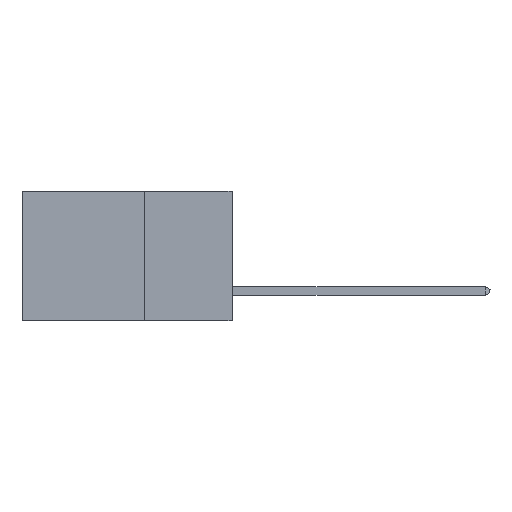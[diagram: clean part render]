
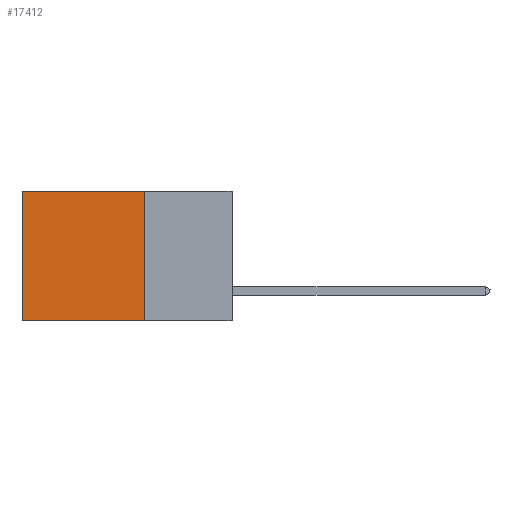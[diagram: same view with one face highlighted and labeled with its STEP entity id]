
A CAD part, left-side view. The second image highlights one B-rep face of the part: STEP entity #17412.
In plain terms, the highlighted planar face has unit normal (-1, 0, 0).
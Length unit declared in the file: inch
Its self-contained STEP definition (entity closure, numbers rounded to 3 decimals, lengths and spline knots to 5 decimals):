
#676 = CARTESIAN_POINT ( 'NONE',  ( 0.2875, 0.25, 0. ) ) ;
#870 = CARTESIAN_POINT ( 'NONE',  ( 0.2875, 0.25, 0. ) ) ;
#1887 = VECTOR ( 'NONE', #19245, 39.37008 ) ;
#3171 = ORIENTED_EDGE ( 'NONE', *, *, #7747, .T. ) ;
#3256 = VERTEX_POINT ( 'NONE', #8707 ) ;
#3292 = VERTEX_POINT ( 'NONE', #13044 ) ;
#3361 = VERTEX_POINT ( 'NONE', #8579 ) ;
#3696 = DIRECTION ( 'NONE',  ( 0., 0., -1. ) ) ;
#4029 = LINE ( 'NONE', #12168, #1887 ) ;
#4373 = AXIS2_PLACEMENT_3D ( 'NONE', #870, #10074, #13257 ) ;
#4620 = EDGE_CURVE ( 'NONE', #3256, #3292, #15008, .T. ) ;
#5298 = DIRECTION ( 'NONE',  ( 0., 1., 0. ) ) ;
#5543 = DIRECTION ( 'NONE',  ( 0., 0., -1. ) ) ;
#6017 = LINE ( 'NONE', #11349, #17293 ) ;
#6098 = EDGE_LOOP ( 'NONE', ( #3171, #15891, #18177, #19231 ) ) ;
#7042 = CARTESIAN_POINT ( 'NONE',  ( 0.2875, 0.25, 0. ) ) ;
#7747 = EDGE_CURVE ( 'NONE', #3361, #13255, #6017, .T. ) ;
#7968 = FACE_OUTER_BOUND ( 'NONE', #6098, .T. ) ;
#8511 = EDGE_CURVE ( 'NONE', #3292, #13255, #4029, .T. ) ;
#8579 = CARTESIAN_POINT ( 'NONE',  ( 0.2875, 0.6, 0. ) ) ;
#8707 = CARTESIAN_POINT ( 'NONE',  ( 0.2875, 0.25, 0. ) ) ;
#10074 = DIRECTION ( 'NONE',  ( 1., 0., 0. ) ) ;
#11349 = CARTESIAN_POINT ( 'NONE',  ( 0.2875, 0.6, 0. ) ) ;
#12168 = CARTESIAN_POINT ( 'NONE',  ( 0.2875, 0.25, -0.37 ) ) ;
#13044 = CARTESIAN_POINT ( 'NONE',  ( 0.2875, 0.25, -0.37 ) ) ;
#13255 = VERTEX_POINT ( 'NONE', #18996 ) ;
#13257 = DIRECTION ( 'NONE',  ( 0., 0., -1. ) ) ;
#13998 = EDGE_CURVE ( 'NONE', #3256, #3361, #17027, .T. ) ;
#15008 = LINE ( 'NONE', #7042, #19341 ) ;
#15891 = ORIENTED_EDGE ( 'NONE', *, *, #8511, .F. ) ;
#17027 = LINE ( 'NONE', #676, #18917 ) ;
#17293 = VECTOR ( 'NONE', #3696, 39.37008 ) ;
#17412 = ADVANCED_FACE ( 'NONE', ( #7968 ), #17647, .F. ) ;
#17647 = PLANE ( 'NONE',  #4373 ) ;
#18177 = ORIENTED_EDGE ( 'NONE', *, *, #4620, .F. ) ;
#18917 = VECTOR ( 'NONE', #5298, 39.37008 ) ;
#18996 = CARTESIAN_POINT ( 'NONE',  ( 0.2875, 0.6, -0.37 ) ) ;
#19231 = ORIENTED_EDGE ( 'NONE', *, *, #13998, .T. ) ;
#19245 = DIRECTION ( 'NONE',  ( 0., 1., 0. ) ) ;
#19341 = VECTOR ( 'NONE', #5543, 39.37008 ) ;
